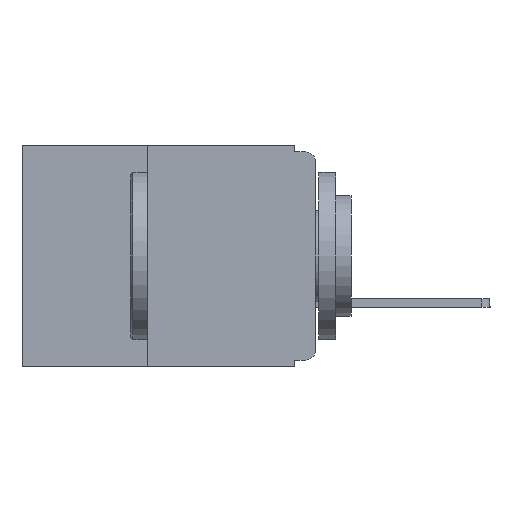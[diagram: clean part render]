
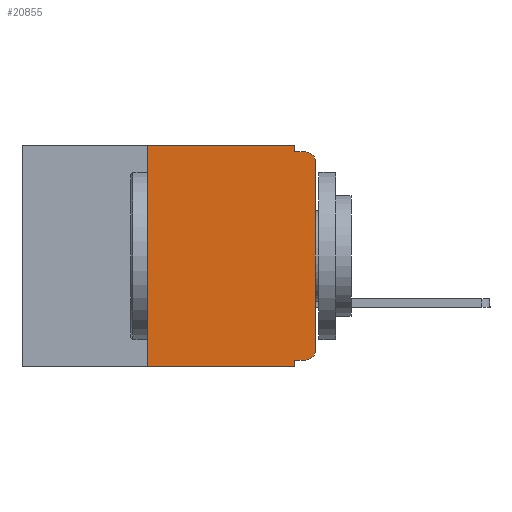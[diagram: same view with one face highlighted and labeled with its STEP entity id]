
A CAD part, left-side view. The second image highlights one B-rep face of the part: STEP entity #20855.
In plain terms, the highlighted planar face has unit normal (-1, 0, 0).
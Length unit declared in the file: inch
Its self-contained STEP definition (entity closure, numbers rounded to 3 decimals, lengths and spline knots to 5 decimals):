
#14 = LINE ( 'NONE', #19717, #8739 ) ;
#443 = VERTEX_POINT ( 'NONE', #13526 ) ;
#461 = AXIS2_PLACEMENT_3D ( 'NONE', #3880, #15334, #5526 ) ;
#626 = ORIENTED_EDGE ( 'NONE', *, *, #19782, .T. ) ;
#645 = VERTEX_POINT ( 'NONE', #21186 ) ;
#794 = DIRECTION ( 'NONE',  ( 1., 0., 0. ) ) ;
#964 = EDGE_CURVE ( 'NONE', #7455, #15792, #16532, .T. ) ;
#1468 = DIRECTION ( 'NONE',  ( 0., -1., 0. ) ) ;
#1797 = ORIENTED_EDGE ( 'NONE', *, *, #11780, .F. ) ;
#1884 = CARTESIAN_POINT ( 'NONE',  ( 0., 0.015, -0.01 ) ) ;
#2073 = ORIENTED_EDGE ( 'NONE', *, *, #2401, .F. ) ;
#2091 = CARTESIAN_POINT ( 'NONE',  ( 0., 0.437, 0. ) ) ;
#2287 = EDGE_CURVE ( 'NONE', #443, #12024, #9265, .T. ) ;
#2393 = DIRECTION ( 'NONE',  ( -1., 0., 0. ) ) ;
#2401 = EDGE_CURVE ( 'NONE', #19553, #7594, #15418, .T. ) ;
#2464 = DIRECTION ( 'NONE',  ( 0., 1., 0. ) ) ;
#2707 = DIRECTION ( 'NONE',  ( 0., 0., 1. ) ) ;
#2708 = ORIENTED_EDGE ( 'NONE', *, *, #18817, .F. ) ;
#3545 = ORIENTED_EDGE ( 'NONE', *, *, #20226, .T. ) ;
#3647 = FACE_OUTER_BOUND ( 'NONE', #15256, .T. ) ;
#3880 = CARTESIAN_POINT ( 'NONE',  ( 0., 0.015, -0.305 ) ) ;
#3927 = VECTOR ( 'NONE', #6511, 39.37008 ) ;
#4176 = ORIENTED_EDGE ( 'NONE', *, *, #19622, .F. ) ;
#4187 = CIRCLE ( 'NONE', #461, 0.015 ) ;
#4258 = VERTEX_POINT ( 'NONE', #13993 ) ;
#4458 = LINE ( 'NONE', #19645, #3927 ) ;
#5042 = ORIENTED_EDGE ( 'NONE', *, *, #2287, .T. ) ;
#5526 = DIRECTION ( 'NONE',  ( 0., 0., -1. ) ) ;
#5696 = VECTOR ( 'NONE', #20430, 39.37008 ) ;
#5732 = DIRECTION ( 'NONE',  ( 0., 0., -1. ) ) ;
#6071 = DIRECTION ( 'NONE',  ( 0., -1., 0. ) ) ;
#6511 = DIRECTION ( 'NONE',  ( 0., 0., -1. ) ) ;
#6955 = CIRCLE ( 'NONE', #14433, 0.015 ) ;
#6977 = LINE ( 'NONE', #12658, #19544 ) ;
#7455 = VERTEX_POINT ( 'NONE', #12921 ) ;
#7594 = VERTEX_POINT ( 'NONE', #1884 ) ;
#8234 = DIRECTION ( 'NONE',  ( 0., 0., -1. ) ) ;
#8739 = VECTOR ( 'NONE', #8234, 39.37008 ) ;
#8746 = VECTOR ( 'NONE', #2707, 39.37008 ) ;
#9027 = DIRECTION ( 'NONE',  ( 0., -1., 0. ) ) ;
#9190 = CARTESIAN_POINT ( 'NONE',  ( 0., 0., -0.01 ) ) ;
#9265 = LINE ( 'NONE', #21211, #8746 ) ;
#10006 = CARTESIAN_POINT ( 'NONE',  ( 0., 0.031, 0. ) ) ;
#10223 = VECTOR ( 'NONE', #2464, 39.37008 ) ;
#10560 = VECTOR ( 'NONE', #9027, 39.37008 ) ;
#10624 = CARTESIAN_POINT ( 'NONE',  ( 0., 0.437, 0. ) ) ;
#10644 = CARTESIAN_POINT ( 'NONE',  ( 0., 0., -0.32 ) ) ;
#11780 = EDGE_CURVE ( 'NONE', #15792, #19553, #4458, .T. ) ;
#11984 = CARTESIAN_POINT ( 'NONE',  ( 0., 0.25, -0.33 ) ) ;
#12004 = EDGE_CURVE ( 'NONE', #4258, #443, #4187, .T. ) ;
#12024 = VERTEX_POINT ( 'NONE', #12040 ) ;
#12040 = CARTESIAN_POINT ( 'NONE',  ( 0., 0., -0.025 ) ) ;
#12108 = AXIS2_PLACEMENT_3D ( 'NONE', #10624, #794, #5732 ) ;
#12204 = CARTESIAN_POINT ( 'NONE',  ( 0., 0.015, -0.025 ) ) ;
#12658 = CARTESIAN_POINT ( 'NONE',  ( 0., 0.437, -0.33 ) ) ;
#12921 = CARTESIAN_POINT ( 'NONE',  ( 0., 0.25, 0. ) ) ;
#13262 = VERTEX_POINT ( 'NONE', #11984 ) ;
#13479 = ORIENTED_EDGE ( 'NONE', *, *, #21063, .F. ) ;
#13495 = CARTESIAN_POINT ( 'NONE',  ( 0., 0.031, -0.32 ) ) ;
#13526 = CARTESIAN_POINT ( 'NONE',  ( 0., 0., -0.305 ) ) ;
#13858 = DIRECTION ( 'NONE',  ( 0., 0., -1. ) ) ;
#13882 = CARTESIAN_POINT ( 'NONE',  ( 0., 0.25, -0.33 ) ) ;
#13993 = CARTESIAN_POINT ( 'NONE',  ( 0., 0.015, -0.32 ) ) ;
#14433 = AXIS2_PLACEMENT_3D ( 'NONE', #12204, #2393, #13858 ) ;
#14790 = LINE ( 'NONE', #10644, #10223 ) ;
#15256 = EDGE_LOOP ( 'NONE', ( #5042, #3545, #2073, #1797, #19514, #4176, #626, #13479, #2708, #18033 ) ) ;
#15323 = CARTESIAN_POINT ( 'NONE',  ( 0., 0.031, -0.01 ) ) ;
#15334 = DIRECTION ( 'NONE',  ( -1., 0., 0. ) ) ;
#15418 = LINE ( 'NONE', #9190, #10560 ) ;
#15546 = PLANE ( 'NONE',  #12108 ) ;
#15792 = VERTEX_POINT ( 'NONE', #10006 ) ;
#16010 = VECTOR ( 'NONE', #1468, 39.37008 ) ;
#16532 = LINE ( 'NONE', #2091, #16010 ) ;
#18033 = ORIENTED_EDGE ( 'NONE', *, *, #12004, .T. ) ;
#18292 = LINE ( 'NONE', #13882, #5696 ) ;
#18677 = VERTEX_POINT ( 'NONE', #13495 ) ;
#18817 = EDGE_CURVE ( 'NONE', #4258, #18677, #14790, .T. ) ;
#19514 = ORIENTED_EDGE ( 'NONE', *, *, #964, .F. ) ;
#19544 = VECTOR ( 'NONE', #6071, 39.37008 ) ;
#19553 = VERTEX_POINT ( 'NONE', #15323 ) ;
#19622 = EDGE_CURVE ( 'NONE', #13262, #7455, #18292, .T. ) ;
#19645 = CARTESIAN_POINT ( 'NONE',  ( 0., 0.031, 0. ) ) ;
#19717 = CARTESIAN_POINT ( 'NONE',  ( 0., 0.031, -0.33 ) ) ;
#19782 = EDGE_CURVE ( 'NONE', #13262, #645, #6977, .T. ) ;
#20226 = EDGE_CURVE ( 'NONE', #12024, #7594, #6955, .T. ) ;
#20430 = DIRECTION ( 'NONE',  ( 0., 0., 1. ) ) ;
#20855 = ADVANCED_FACE ( 'NONE', ( #3647 ), #15546, .F. ) ;
#21063 = EDGE_CURVE ( 'NONE', #18677, #645, #14, .T. ) ;
#21186 = CARTESIAN_POINT ( 'NONE',  ( 0., 0.031, -0.33 ) ) ;
#21211 = CARTESIAN_POINT ( 'NONE',  ( 0., 0., 0. ) ) ;
